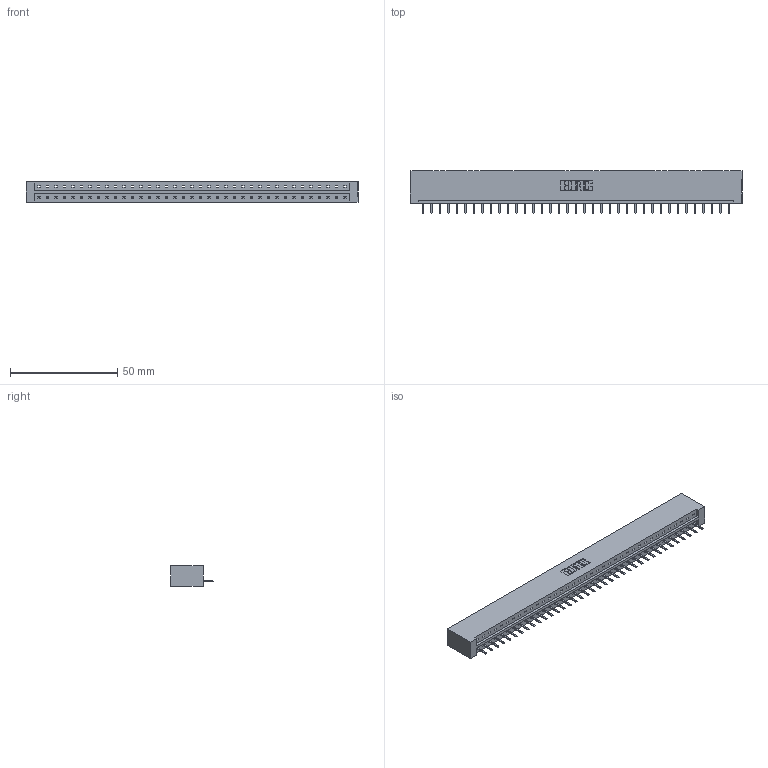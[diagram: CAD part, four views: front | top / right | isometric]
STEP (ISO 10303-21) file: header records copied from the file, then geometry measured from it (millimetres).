
FILE_DESCRIPTION (( 'STEP AP203' ), '1' );
FILE_NAME ('833-037-520-101.STEP', '2020-06-03T04:38:40', ( '' ), ( '' ), 'SwSTEP 2.0', 'SolidWorks 2020', '' );
FILE_SCHEMA (( 'CONFIG_CONTROL_DESIGN' ));
Length unit declared in the file: inch
Products named in the file (3): 345-292-001_345-293-120; 833-037-520-101; 833 Part_Lugless
Assembly tree (38 placements, depth 2):
  833-037-520-101
    833 Part_Lugless
    345-292-001_345-293-120  x37
Bounding box: 154.86 x 20.02 x 9.4 mm (x, y, z)
Volume: 16047 mm3; surface area: 16913 mm2
Topology: 38 solids, 38 shells, 2400 faces, 7095 edges, 4630 vertices
Faces by surface type: plane 1694, cylinder 706
Entity records: 23103 total; most frequent: CARTESIAN_POINT 4005, ORIENTED_EDGE 3966, DIRECTION 3369, EDGE_CURVE 1983, VECTOR 1859, LINE 1859, VERTEX_POINT 1318, AXIS2_PLACEMENT_3D 755
